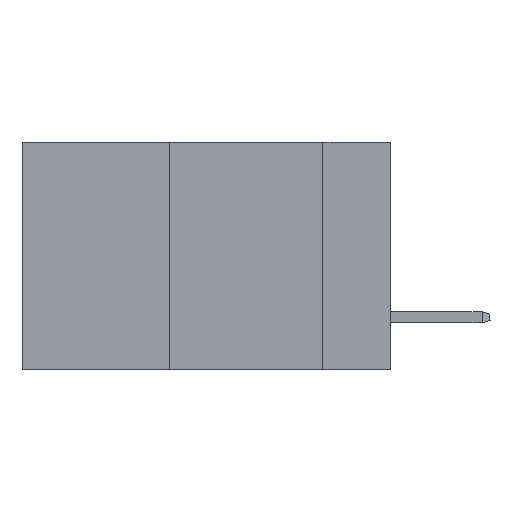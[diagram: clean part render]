
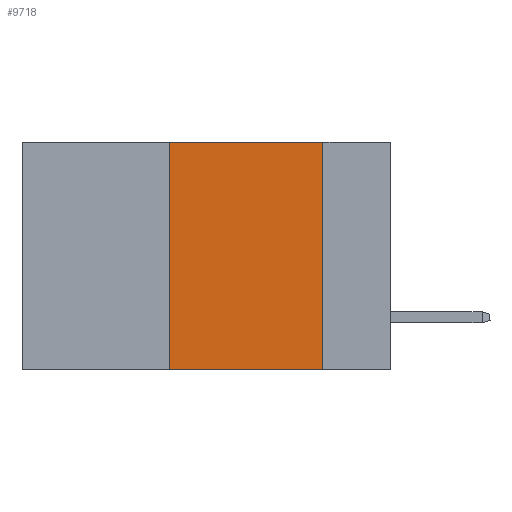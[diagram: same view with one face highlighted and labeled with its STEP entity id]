
A CAD part, left-side view. The second image highlights one B-rep face of the part: STEP entity #9718.
In plain terms, the highlighted planar face has unit normal (-1, 0, 0).
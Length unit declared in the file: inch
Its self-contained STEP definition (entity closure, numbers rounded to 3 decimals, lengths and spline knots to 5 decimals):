
#1415 = CARTESIAN_POINT ( 'NONE',  ( 0., 0.6, -0.37 ) ) ;
#1716 = VERTEX_POINT ( 'NONE', #18129 ) ;
#2159 = VECTOR ( 'NONE', #26185, 39.37008 ) ;
#2548 = ORIENTED_EDGE ( 'NONE', *, *, #19083, .F. ) ;
#3071 = DIRECTION ( 'NONE',  ( 0., 0., -1. ) ) ;
#6965 = PLANE ( 'NONE',  #8500 ) ;
#7931 = DIRECTION ( 'NONE',  ( 0., -1., 0. ) ) ;
#8500 = AXIS2_PLACEMENT_3D ( 'NONE', #11219, #23170, #3071 ) ;
#9718 = ADVANCED_FACE ( 'NONE', ( #23694 ), #6965, .F. ) ;
#11064 = LINE ( 'NONE', #25931, #19661 ) ;
#11219 = CARTESIAN_POINT ( 'NONE',  ( 0., 0.6, 0. ) ) ;
#11334 = DIRECTION ( 'NONE',  ( 0., 0., 1. ) ) ;
#11465 = VERTEX_POINT ( 'NONE', #13258 ) ;
#11839 = VERTEX_POINT ( 'NONE', #15698 ) ;
#11947 = ORIENTED_EDGE ( 'NONE', *, *, #19152, .F. ) ;
#12025 = CARTESIAN_POINT ( 'NONE',  ( 0., 0.11, 0. ) ) ;
#12110 = EDGE_CURVE ( 'NONE', #25166, #1716, #23205, .T. ) ;
#12617 = ORIENTED_EDGE ( 'NONE', *, *, #18874, .F. ) ;
#13258 = CARTESIAN_POINT ( 'NONE',  ( 0., 0.11, 0. ) ) ;
#15698 = CARTESIAN_POINT ( 'NONE',  ( 0., 0.36, 0. ) ) ;
#16602 = VECTOR ( 'NONE', #17759, 39.37008 ) ;
#17149 = LINE ( 'NONE', #19589, #25345 ) ;
#17759 = DIRECTION ( 'NONE',  ( 0., -1., 0. ) ) ;
#18129 = CARTESIAN_POINT ( 'NONE',  ( 0., 0.11, -0.37 ) ) ;
#18874 = EDGE_CURVE ( 'NONE', #25166, #11839, #17149, .T. ) ;
#19083 = EDGE_CURVE ( 'NONE', #11839, #11465, #11064, .T. ) ;
#19152 = EDGE_CURVE ( 'NONE', #11465, #1716, #22441, .T. ) ;
#19589 = CARTESIAN_POINT ( 'NONE',  ( 0., 0.36, 0. ) ) ;
#19661 = VECTOR ( 'NONE', #7931, 39.37008 ) ;
#21571 = CARTESIAN_POINT ( 'NONE',  ( 0., 0.36, -0.37 ) ) ;
#22123 = EDGE_LOOP ( 'NONE', ( #11947, #2548, #12617, #25232 ) ) ;
#22441 = LINE ( 'NONE', #12025, #2159 ) ;
#23170 = DIRECTION ( 'NONE',  ( 1., 0., 0. ) ) ;
#23205 = LINE ( 'NONE', #1415, #16602 ) ;
#23694 = FACE_OUTER_BOUND ( 'NONE', #22123, .T. ) ;
#25166 = VERTEX_POINT ( 'NONE', #21571 ) ;
#25232 = ORIENTED_EDGE ( 'NONE', *, *, #12110, .T. ) ;
#25345 = VECTOR ( 'NONE', #11334, 39.37008 ) ;
#25931 = CARTESIAN_POINT ( 'NONE',  ( 0., 0.6, 0. ) ) ;
#26185 = DIRECTION ( 'NONE',  ( 0., 0., -1. ) ) ;
